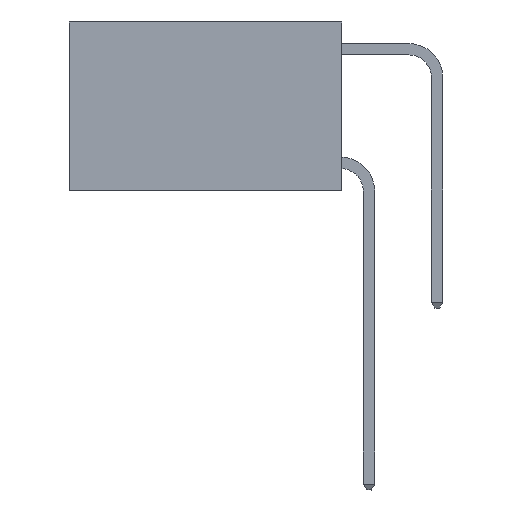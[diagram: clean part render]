
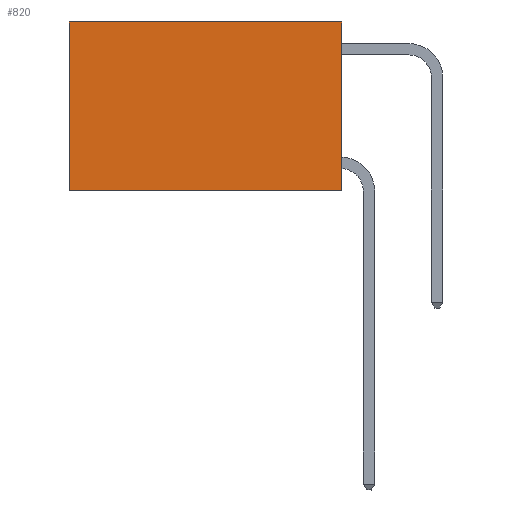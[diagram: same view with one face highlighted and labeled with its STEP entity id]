
A CAD part, left-side view. The second image highlights one B-rep face of the part: STEP entity #820.
In plain terms, the highlighted planar face has unit normal (-1, 0, 0).
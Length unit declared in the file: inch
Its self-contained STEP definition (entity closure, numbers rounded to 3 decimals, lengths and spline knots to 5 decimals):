
#820 = ADVANCED_FACE ( 'NONE', ( #9221 ), #1995, .F. ) ;
#1472 = VECTOR ( 'NONE', #6663, 39.37008 ) ;
#1614 = VERTEX_POINT ( 'NONE', #3506 ) ;
#1773 = EDGE_CURVE ( 'NONE', #11866, #3356, #9493, .T. ) ;
#1995 = PLANE ( 'NONE',  #4376 ) ;
#2374 = VERTEX_POINT ( 'NONE', #5158 ) ;
#2782 = DIRECTION ( 'NONE',  ( 0., 0., -1. ) ) ;
#3356 = VERTEX_POINT ( 'NONE', #5982 ) ;
#3506 = CARTESIAN_POINT ( 'NONE',  ( 0.2625, 0., -0.37 ) ) ;
#3952 = DIRECTION ( 'NONE',  ( 0., 0., -1. ) ) ;
#4376 = AXIS2_PLACEMENT_3D ( 'NONE', #6897, #9712, #3952 ) ;
#4458 = ORIENTED_EDGE ( 'NONE', *, *, #9808, .F. ) ;
#4684 = DIRECTION ( 'NONE',  ( 0., 1., 0. ) ) ;
#4950 = EDGE_LOOP ( 'NONE', ( #8772, #8263, #4458, #9698 ) ) ;
#5119 = VECTOR ( 'NONE', #4684, 39.37008 ) ;
#5158 = CARTESIAN_POINT ( 'NONE',  ( 0.2625, 0.6, -0.37 ) ) ;
#5291 = EDGE_CURVE ( 'NONE', #1614, #2374, #5784, .T. ) ;
#5377 = CARTESIAN_POINT ( 'NONE',  ( 0.2625, 0., 0. ) ) ;
#5784 = LINE ( 'NONE', #11288, #5119 ) ;
#5982 = CARTESIAN_POINT ( 'NONE',  ( 0.2625, 0.6, 0. ) ) ;
#6436 = LINE ( 'NONE', #9540, #11040 ) ;
#6663 = DIRECTION ( 'NONE',  ( 0., 1., 0. ) ) ;
#6897 = CARTESIAN_POINT ( 'NONE',  ( 0.2625, 0., 0. ) ) ;
#8263 = ORIENTED_EDGE ( 'NONE', *, *, #5291, .F. ) ;
#8772 = ORIENTED_EDGE ( 'NONE', *, *, #10446, .T. ) ;
#9221 = FACE_OUTER_BOUND ( 'NONE', #4950, .T. ) ;
#9392 = LINE ( 'NONE', #10649, #11449 ) ;
#9461 = CARTESIAN_POINT ( 'NONE',  ( 0.2625, 0., 0. ) ) ;
#9493 = LINE ( 'NONE', #9461, #1472 ) ;
#9540 = CARTESIAN_POINT ( 'NONE',  ( 0.2625, 0.6, 0. ) ) ;
#9698 = ORIENTED_EDGE ( 'NONE', *, *, #1773, .T. ) ;
#9712 = DIRECTION ( 'NONE',  ( 1., 0., 0. ) ) ;
#9808 = EDGE_CURVE ( 'NONE', #11866, #1614, #9392, .T. ) ;
#10446 = EDGE_CURVE ( 'NONE', #3356, #2374, #6436, .T. ) ;
#10649 = CARTESIAN_POINT ( 'NONE',  ( 0.2625, 0., 0. ) ) ;
#11040 = VECTOR ( 'NONE', #2782, 39.37008 ) ;
#11288 = CARTESIAN_POINT ( 'NONE',  ( 0.2625, 0., -0.37 ) ) ;
#11449 = VECTOR ( 'NONE', #11533, 39.37008 ) ;
#11533 = DIRECTION ( 'NONE',  ( 0., 0., -1. ) ) ;
#11866 = VERTEX_POINT ( 'NONE', #5377 ) ;
